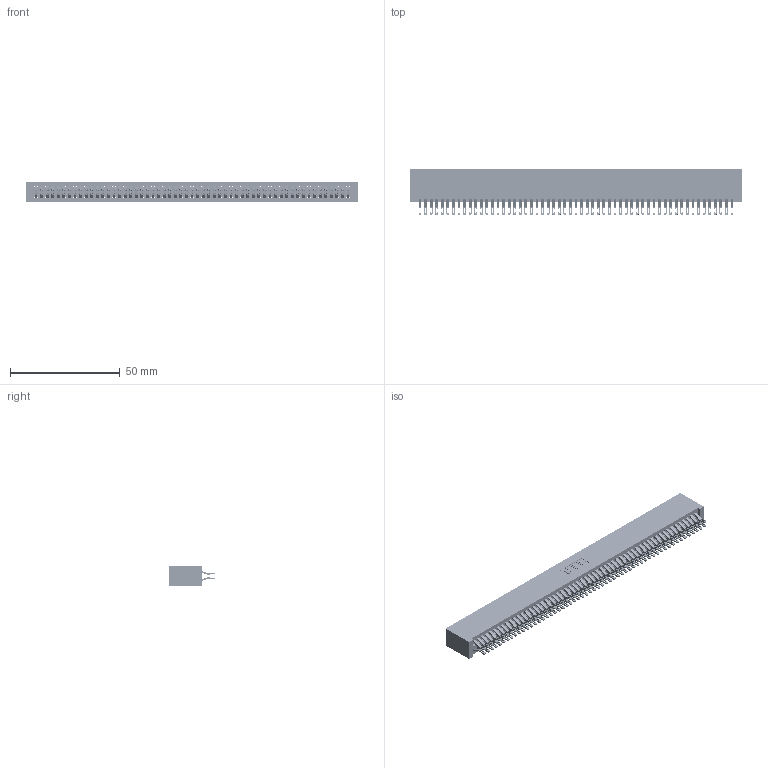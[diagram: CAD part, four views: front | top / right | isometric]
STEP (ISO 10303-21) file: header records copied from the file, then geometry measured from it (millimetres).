
FILE_DESCRIPTION (( 'STEP AP203' ), '1' );
FILE_NAME ('345-114-555-201.STEP', '2019-11-05T12:06:34', ( '' ), ( '' ), 'SwSTEP 2.0', 'SolidWorks 2016', '' );
FILE_SCHEMA (( 'CONFIG_CONTROL_DESIGN' ));
Length unit declared in the file: inch
Products named in the file (3): 345-114-555-201; 345 Part_No Mounting Lugs; 345-292-001_555 Tail
Assembly tree (115 placements, depth 2):
  345-114-555-201
    345 Part_No Mounting Lugs
    345-292-001_555 Tail  x114
Bounding box: 151.38 x 21.13 x 9.4 mm (x, y, z)
Volume: 15791.4 mm3; surface area: 25086.2 mm2
Topology: 115 solids, 115 shells, 6502 faces, 20495 edges, 13662 vertices
Faces by surface type: plane 3610, cylinder 2892
Entity records: 42753 total; most frequent: CARTESIAN_POINT 7186, ORIENTED_EDGE 7090, DIRECTION 6281, EDGE_CURVE 3545, LINE 3173, VECTOR 3173, VERTEX_POINT 2362, AXIS2_PLACEMENT_3D 1554
